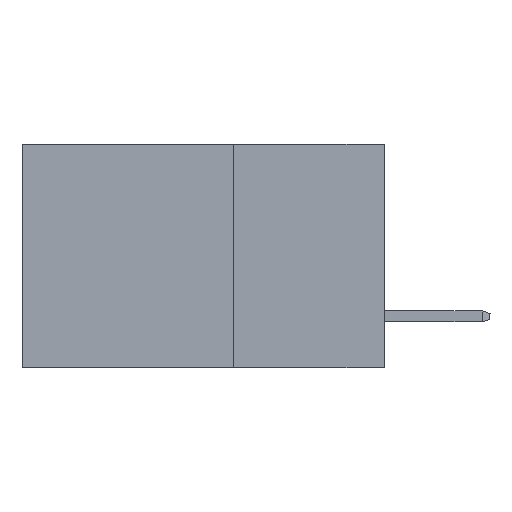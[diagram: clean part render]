
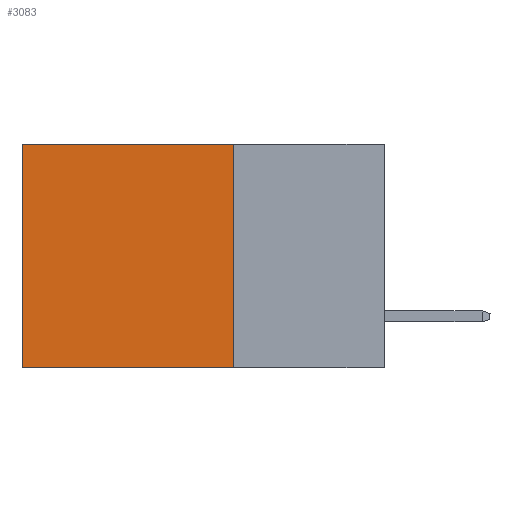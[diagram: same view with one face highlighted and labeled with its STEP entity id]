
A CAD part, left-side view. The second image highlights one B-rep face of the part: STEP entity #3083.
In plain terms, the highlighted planar face has unit normal (-1, 0, 0).
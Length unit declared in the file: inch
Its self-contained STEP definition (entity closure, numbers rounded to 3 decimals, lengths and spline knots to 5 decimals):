
#18 = AXIS2_PLACEMENT_3D ( 'NONE', #3951, #1707, #7001 ) ;
#123 = PLANE ( 'NONE',  #18 ) ;
#378 = LINE ( 'NONE', #8939, #6249 ) ;
#421 = DIRECTION ( 'NONE',  ( 0., 0., -1. ) ) ;
#1191 = EDGE_CURVE ( 'NONE', #10040, #2974, #378, .T. ) ;
#1258 = CARTESIAN_POINT ( 'NONE',  ( 0.2615, 0.6, 0. ) ) ;
#1454 = VERTEX_POINT ( 'NONE', #6424 ) ;
#1707 = DIRECTION ( 'NONE',  ( 1., 0., 0. ) ) ;
#1841 = CARTESIAN_POINT ( 'NONE',  ( 0.2615, 0.25, -0.37 ) ) ;
#2391 = ORIENTED_EDGE ( 'NONE', *, *, #1191, .T. ) ;
#2523 = FACE_OUTER_BOUND ( 'NONE', #5717, .T. ) ;
#2895 = LINE ( 'NONE', #6002, #4033 ) ;
#2974 = VERTEX_POINT ( 'NONE', #4001 ) ;
#2990 = CARTESIAN_POINT ( 'NONE',  ( 0.2615, 0.25, 0. ) ) ;
#3083 = ADVANCED_FACE ( 'NONE', ( #2523 ), #123, .F. ) ;
#3144 = DIRECTION ( 'NONE',  ( 0., 1., 0. ) ) ;
#3190 = DIRECTION ( 'NONE',  ( 0., 1., 0. ) ) ;
#3194 = CARTESIAN_POINT ( 'NONE',  ( 0.2615, 0.25, 0. ) ) ;
#3951 = CARTESIAN_POINT ( 'NONE',  ( 0.2615, 0.25, -0.37 ) ) ;
#4001 = CARTESIAN_POINT ( 'NONE',  ( 0.2615, 0.6, -0.37 ) ) ;
#4033 = VECTOR ( 'NONE', #3190, 39.37008 ) ;
#4229 = ORIENTED_EDGE ( 'NONE', *, *, #8833, .F. ) ;
#5370 = ORIENTED_EDGE ( 'NONE', *, *, #6265, .F. ) ;
#5704 = DIRECTION ( 'NONE',  ( 0., 0., -1. ) ) ;
#5717 = EDGE_LOOP ( 'NONE', ( #2391, #5370, #4229, #8634 ) ) ;
#6002 = CARTESIAN_POINT ( 'NONE',  ( 0.2615, 0.25, -0.37 ) ) ;
#6249 = VECTOR ( 'NONE', #421, 39.37008 ) ;
#6265 = EDGE_CURVE ( 'NONE', #1454, #2974, #2895, .T. ) ;
#6311 = LINE ( 'NONE', #1841, #8136 ) ;
#6424 = CARTESIAN_POINT ( 'NONE',  ( 0.2615, 0.25, -0.37 ) ) ;
#7001 = DIRECTION ( 'NONE',  ( 0., 0., -1. ) ) ;
#7806 = VECTOR ( 'NONE', #3144, 39.37008 ) ;
#8007 = VERTEX_POINT ( 'NONE', #2990 ) ;
#8136 = VECTOR ( 'NONE', #5704, 39.37008 ) ;
#8634 = ORIENTED_EDGE ( 'NONE', *, *, #9218, .T. ) ;
#8833 = EDGE_CURVE ( 'NONE', #8007, #1454, #6311, .T. ) ;
#8939 = CARTESIAN_POINT ( 'NONE',  ( 0.2615, 0.6, -0.37 ) ) ;
#9218 = EDGE_CURVE ( 'NONE', #8007, #10040, #9371, .T. ) ;
#9371 = LINE ( 'NONE', #3194, #7806 ) ;
#10040 = VERTEX_POINT ( 'NONE', #1258 ) ;
